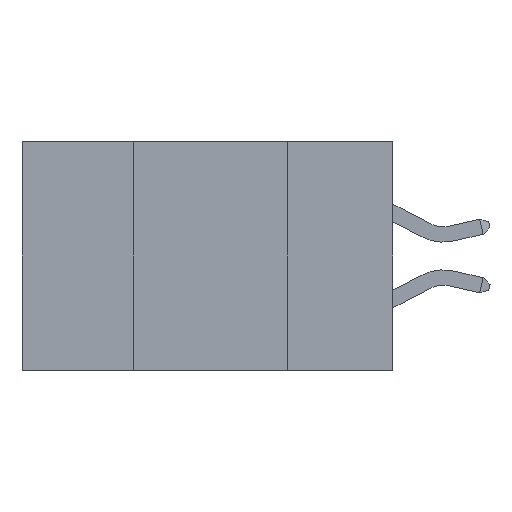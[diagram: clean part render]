
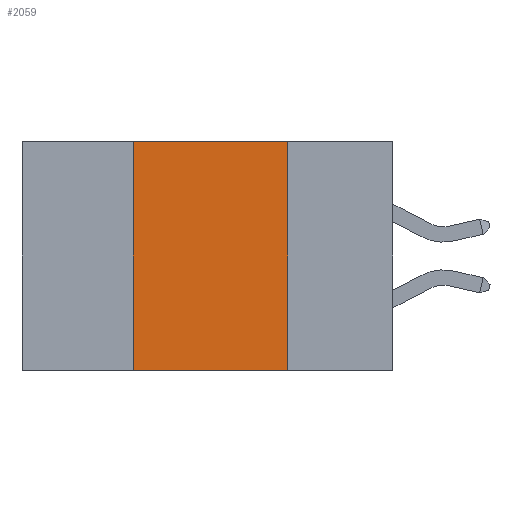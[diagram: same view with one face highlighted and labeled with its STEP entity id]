
A CAD part, left-side view. The second image highlights one B-rep face of the part: STEP entity #2059.
In plain terms, the highlighted planar face has unit normal (-1, 0, 0).
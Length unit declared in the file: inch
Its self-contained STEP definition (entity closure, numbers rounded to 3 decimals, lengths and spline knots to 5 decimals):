
#300 = CARTESIAN_POINT ( 'NONE',  ( 0., 0.42, 0. ) ) ;
#801 = VERTEX_POINT ( 'NONE', #9275 ) ;
#1189 = LINE ( 'NONE', #300, #8636 ) ;
#1457 = EDGE_CURVE ( 'NONE', #8618, #801, #10242, .T. ) ;
#1549 = ORIENTED_EDGE ( 'NONE', *, *, #1457, .T. ) ;
#1904 = EDGE_CURVE ( 'NONE', #8618, #7604, #1189, .T. ) ;
#1928 = FACE_OUTER_BOUND ( 'NONE', #4274, .T. ) ;
#2059 = ADVANCED_FACE ( 'NONE', ( #1928 ), #9565, .F. ) ;
#2777 = DIRECTION ( 'NONE',  ( 0., 0., 1. ) ) ;
#2850 = VECTOR ( 'NONE', #3844, 39.37008 ) ;
#2945 = VECTOR ( 'NONE', #6693, 39.37008 ) ;
#3342 = AXIS2_PLACEMENT_3D ( 'NONE', #3614, #8438, #5082 ) ;
#3614 = CARTESIAN_POINT ( 'NONE',  ( 0., 0.6, 0. ) ) ;
#3844 = DIRECTION ( 'NONE',  ( 0., -1., 0. ) ) ;
#4073 = EDGE_CURVE ( 'NONE', #10086, #801, #8866, .T. ) ;
#4103 = CARTESIAN_POINT ( 'NONE',  ( 0., 0.6, -0.37 ) ) ;
#4274 = EDGE_LOOP ( 'NONE', ( #7098, #7016, #9053, #1549 ) ) ;
#4918 = CARTESIAN_POINT ( 'NONE',  ( 0., 0.42, 0. ) ) ;
#4989 = CARTESIAN_POINT ( 'NONE',  ( 0., 0.42, -0.37 ) ) ;
#5082 = DIRECTION ( 'NONE',  ( 0., 0., -1. ) ) ;
#5358 = CARTESIAN_POINT ( 'NONE',  ( 0., 0.17, 0. ) ) ;
#5790 = VECTOR ( 'NONE', #8790, 39.37008 ) ;
#6693 = DIRECTION ( 'NONE',  ( 0., 0., -1. ) ) ;
#7016 = ORIENTED_EDGE ( 'NONE', *, *, #8976, .F. ) ;
#7098 = ORIENTED_EDGE ( 'NONE', *, *, #4073, .F. ) ;
#7604 = VERTEX_POINT ( 'NONE', #4918 ) ;
#8438 = DIRECTION ( 'NONE',  ( 1., 0., 0. ) ) ;
#8618 = VERTEX_POINT ( 'NONE', #4989 ) ;
#8636 = VECTOR ( 'NONE', #2777, 39.37008 ) ;
#8790 = DIRECTION ( 'NONE',  ( 0., -1., 0. ) ) ;
#8866 = LINE ( 'NONE', #11432, #2945 ) ;
#8976 = EDGE_CURVE ( 'NONE', #7604, #10086, #9083, .T. ) ;
#9053 = ORIENTED_EDGE ( 'NONE', *, *, #1904, .F. ) ;
#9083 = LINE ( 'NONE', #10612, #5790 ) ;
#9275 = CARTESIAN_POINT ( 'NONE',  ( 0., 0.17, -0.37 ) ) ;
#9565 = PLANE ( 'NONE',  #3342 ) ;
#10086 = VERTEX_POINT ( 'NONE', #5358 ) ;
#10242 = LINE ( 'NONE', #4103, #2850 ) ;
#10612 = CARTESIAN_POINT ( 'NONE',  ( 0., 0.6, 0. ) ) ;
#11432 = CARTESIAN_POINT ( 'NONE',  ( 0., 0.17, 0. ) ) ;
